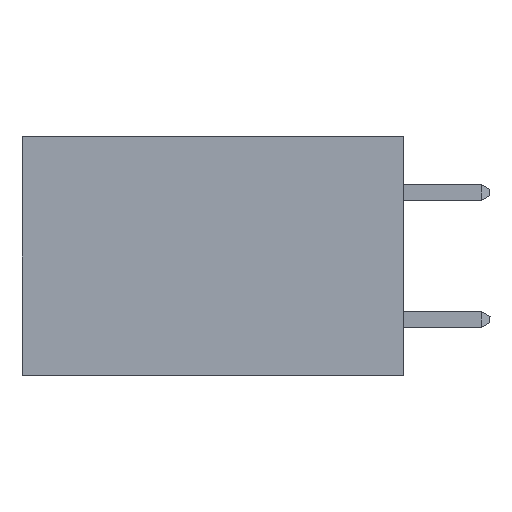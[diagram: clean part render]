
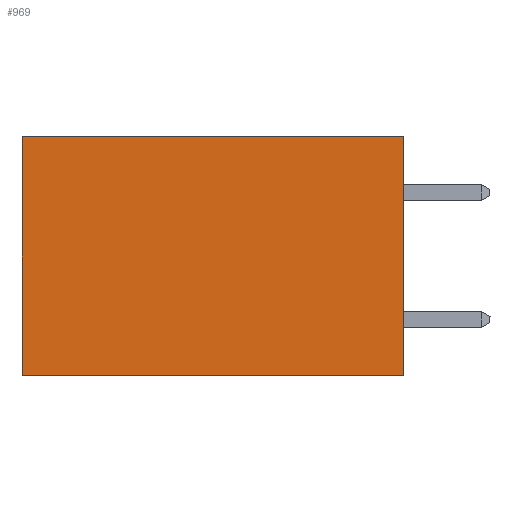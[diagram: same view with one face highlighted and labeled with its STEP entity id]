
A CAD part, left-side view. The second image highlights one B-rep face of the part: STEP entity #969.
In plain terms, the highlighted planar face has unit normal (-1, 0, 0).
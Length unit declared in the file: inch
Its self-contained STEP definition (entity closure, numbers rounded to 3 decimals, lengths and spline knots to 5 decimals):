
#140 = VERTEX_POINT ( 'NONE', #12569 ) ;
#926 = LINE ( 'NONE', #2586, #18203 ) ;
#969 = ADVANCED_FACE ( 'NONE', ( #1534 ), #9687, .F. ) ;
#1534 = FACE_OUTER_BOUND ( 'NONE', #10022, .T. ) ;
#1884 = CARTESIAN_POINT ( 'NONE',  ( 0.2875, 0., -0.375 ) ) ;
#2167 = CARTESIAN_POINT ( 'NONE',  ( 0.2875, 0., -0.375 ) ) ;
#2586 = CARTESIAN_POINT ( 'NONE',  ( 0.2875, 0., -0.375 ) ) ;
#2914 = EDGE_CURVE ( 'NONE', #9295, #14592, #6460, .T. ) ;
#3017 = ORIENTED_EDGE ( 'NONE', *, *, #17131, .F. ) ;
#3042 = ORIENTED_EDGE ( 'NONE', *, *, #2914, .T. ) ;
#5452 = CARTESIAN_POINT ( 'NONE',  ( 0.2875, 0.6, -0.375 ) ) ;
#5512 = DIRECTION ( 'NONE',  ( 0., 1., 0. ) ) ;
#5987 = CARTESIAN_POINT ( 'NONE',  ( 0.2875, 0., 0. ) ) ;
#6460 = LINE ( 'NONE', #6822, #14586 ) ;
#6822 = CARTESIAN_POINT ( 'NONE',  ( 0.2875, 0., 0. ) ) ;
#7223 = DIRECTION ( 'NONE',  ( 0., 0., -1. ) ) ;
#7257 = DIRECTION ( 'NONE',  ( 0., 0., -1. ) ) ;
#7915 = DIRECTION ( 'NONE',  ( 0., 0., -1. ) ) ;
#7959 = EDGE_CURVE ( 'NONE', #14592, #140, #20167, .T. ) ;
#8698 = ORIENTED_EDGE ( 'NONE', *, *, #7959, .T. ) ;
#8778 = LINE ( 'NONE', #2167, #16130 ) ;
#9295 = VERTEX_POINT ( 'NONE', #5987 ) ;
#9436 = VECTOR ( 'NONE', #7257, 39.37008 ) ;
#9687 = PLANE ( 'NONE',  #10399 ) ;
#10022 = EDGE_LOOP ( 'NONE', ( #8698, #3017, #10233, #3042 ) ) ;
#10233 = ORIENTED_EDGE ( 'NONE', *, *, #17993, .F. ) ;
#10399 = AXIS2_PLACEMENT_3D ( 'NONE', #11077, #16267, #7915 ) ;
#11077 = CARTESIAN_POINT ( 'NONE',  ( 0.2875, 0., -0.375 ) ) ;
#12569 = CARTESIAN_POINT ( 'NONE',  ( 0.2875, 0.6, -0.375 ) ) ;
#13476 = VERTEX_POINT ( 'NONE', #1884 ) ;
#13963 = CARTESIAN_POINT ( 'NONE',  ( 0.2875, 0.6, 0. ) ) ;
#14586 = VECTOR ( 'NONE', #15364, 39.37008 ) ;
#14592 = VERTEX_POINT ( 'NONE', #13963 ) ;
#15364 = DIRECTION ( 'NONE',  ( 0., 1., 0. ) ) ;
#16130 = VECTOR ( 'NONE', #5512, 39.37008 ) ;
#16267 = DIRECTION ( 'NONE',  ( 1., 0., 0. ) ) ;
#17131 = EDGE_CURVE ( 'NONE', #13476, #140, #8778, .T. ) ;
#17993 = EDGE_CURVE ( 'NONE', #9295, #13476, #926, .T. ) ;
#18203 = VECTOR ( 'NONE', #7223, 39.37008 ) ;
#20167 = LINE ( 'NONE', #5452, #9436 ) ;
